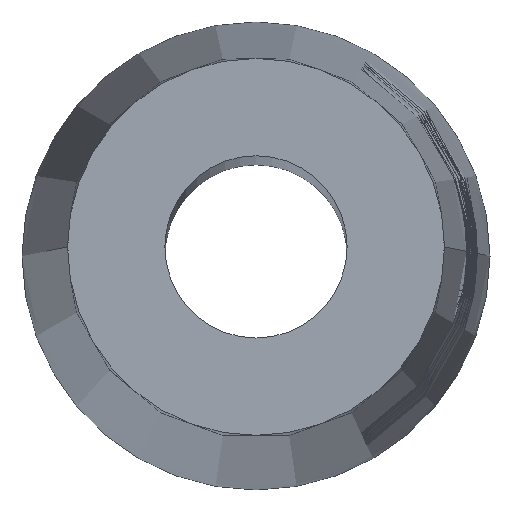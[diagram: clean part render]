
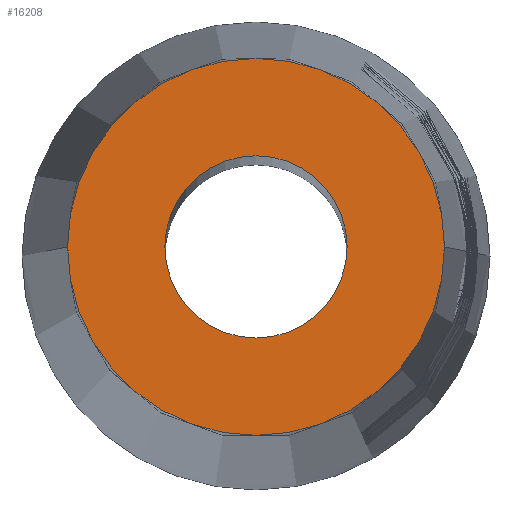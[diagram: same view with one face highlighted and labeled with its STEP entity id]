
A CAD part, top view. The second image highlights one B-rep face of the part: STEP entity #16208.
In plain terms, the highlighted planar face has unit normal (0, 0, 1).
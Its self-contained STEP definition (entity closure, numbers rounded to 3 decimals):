
#311 = DIRECTION ( 'NONE',  ( 1., 0., 0. ) ) ;
#531 = ORIENTED_EDGE ( 'NONE', *, *, #18240, .T. ) ;
#656 = EDGE_LOOP ( 'NONE', ( #15855, #531 ) ) ;
#1272 = DIRECTION ( 'NONE',  ( 1., 0., 0. ) ) ;
#1921 = CARTESIAN_POINT ( 'NONE',  ( 2.794, 0., 160. ) ) ;
#3078 = CIRCLE ( 'NONE', #4809, 2.794 ) ;
#3161 = ORIENTED_EDGE ( 'NONE', *, *, #12587, .F. ) ;
#3920 = CARTESIAN_POINT ( 'NONE',  ( -5.779, 0., 160. ) ) ;
#4064 = EDGE_CURVE ( 'NONE', #13819, #10737, #11026, .T. ) ;
#4166 = CARTESIAN_POINT ( 'NONE',  ( -2.794, 0., 160. ) ) ;
#4543 = VERTEX_POINT ( 'NONE', #3920 ) ;
#4809 = AXIS2_PLACEMENT_3D ( 'NONE', #19545, #10457, #1272 ) ;
#5216 = AXIS2_PLACEMENT_3D ( 'NONE', #14529, #5397, #16095 ) ;
#5397 = DIRECTION ( 'NONE',  ( 0., 0., 1. ) ) ;
#5793 = ORIENTED_EDGE ( 'NONE', *, *, #4064, .F. ) ;
#6427 = DIRECTION ( 'NONE',  ( 0., 0., 1. ) ) ;
#7634 = EDGE_CURVE ( 'NONE', #14326, #4543, #18916, .T. ) ;
#8165 = CARTESIAN_POINT ( 'NONE',  ( 0., 0., 160. ) ) ;
#8695 = FACE_BOUND ( 'NONE', #15261, .T. ) ;
#9479 = DIRECTION ( 'NONE',  ( 0., 0., 1. ) ) ;
#9705 = DIRECTION ( 'NONE',  ( 1., 0., 0. ) ) ;
#9925 = CARTESIAN_POINT ( 'NONE',  ( 5.779, 0., 160. ) ) ;
#10191 = AXIS2_PLACEMENT_3D ( 'NONE', #15571, #6427, #17136 ) ;
#10457 = DIRECTION ( 'NONE',  ( 0., 0., 1. ) ) ;
#10737 = VERTEX_POINT ( 'NONE', #4166 ) ;
#11026 = CIRCLE ( 'NONE', #16920, 2.794 ) ;
#12587 = EDGE_CURVE ( 'NONE', #10737, #13819, #3078, .T. ) ;
#12806 = FACE_OUTER_BOUND ( 'NONE', #656, .T. ) ;
#13011 = PLANE ( 'NONE',  #5216 ) ;
#13819 = VERTEX_POINT ( 'NONE', #1921 ) ;
#14012 = AXIS2_PLACEMENT_3D ( 'NONE', #8165, #18852, #9705 ) ;
#14326 = VERTEX_POINT ( 'NONE', #9925 ) ;
#14529 = CARTESIAN_POINT ( 'NONE',  ( 0., 0., 160. ) ) ;
#15261 = EDGE_LOOP ( 'NONE', ( #5793, #3161 ) ) ;
#15571 = CARTESIAN_POINT ( 'NONE',  ( 0., 0., 160. ) ) ;
#15855 = ORIENTED_EDGE ( 'NONE', *, *, #7634, .T. ) ;
#16095 = DIRECTION ( 'NONE',  ( 1., 0., 0. ) ) ;
#16208 = ADVANCED_FACE ( 'NONE', ( #8695, #12806 ), #13011, .T. ) ;
#16920 = AXIS2_PLACEMENT_3D ( 'NONE', #18635, #9479, #311 ) ;
#17136 = DIRECTION ( 'NONE',  ( 1., 0., 0. ) ) ;
#17787 = CIRCLE ( 'NONE', #10191, 5.779 ) ;
#18240 = EDGE_CURVE ( 'NONE', #4543, #14326, #17787, .T. ) ;
#18635 = CARTESIAN_POINT ( 'NONE',  ( 0., 0., 160. ) ) ;
#18852 = DIRECTION ( 'NONE',  ( 0., 0., 1. ) ) ;
#18916 = CIRCLE ( 'NONE', #14012, 5.779 ) ;
#19545 = CARTESIAN_POINT ( 'NONE',  ( 0., 0., 160. ) ) ;
